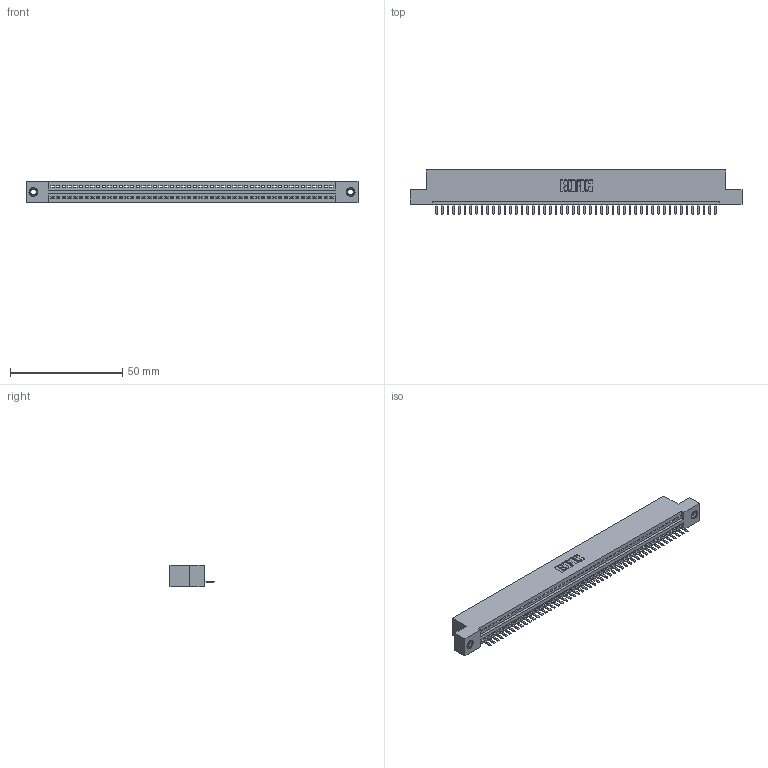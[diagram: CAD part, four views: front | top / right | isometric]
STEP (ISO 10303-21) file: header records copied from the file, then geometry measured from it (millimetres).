
FILE_DESCRIPTION (( 'STEP AP203' ), '1' );
FILE_NAME ('345-050-520-107.STEP', '2019-10-09T10:34:52', ( '' ), ( '' ), 'SwSTEP 2.0', 'SolidWorks 2016', '' );
FILE_SCHEMA (( 'CONFIG_CONTROL_DESIGN' ));
Length unit declared in the file: inch
Products named in the file (4): 345-050-520-107; 345-292-001_345-293-120; 345 Part_Flush Mounting Lugs - 0.156 Dia-TI; 345-250-001_345-250-005-103
Assembly tree (53 placements, depth 2):
  345-050-520-107
    345 Part_Flush Mounting Lugs - 0.156 Dia-TI
    345-292-001_345-293-120  x50
    345-250-001_345-250-005-103  x2
Bounding box: 148.21 x 19.68 x 9.4 mm (x, y, z)
Volume: 13985.2 mm3; surface area: 18255.9 mm2
Topology: 53 solids, 53 shells, 3286 faces, 9677 edges, 6310 vertices
Faces by surface type: plane 2212, cylinder 1058, cone 12, torus 4
Entity records: 37854 total; most frequent: CARTESIAN_POINT 6549, ORIENTED_EDGE 6514, DIRECTION 5723, EDGE_CURVE 3257, VECTOR 2901, LINE 2901, VERTEX_POINT 2164, AXIS2_PLACEMENT_3D 1411
